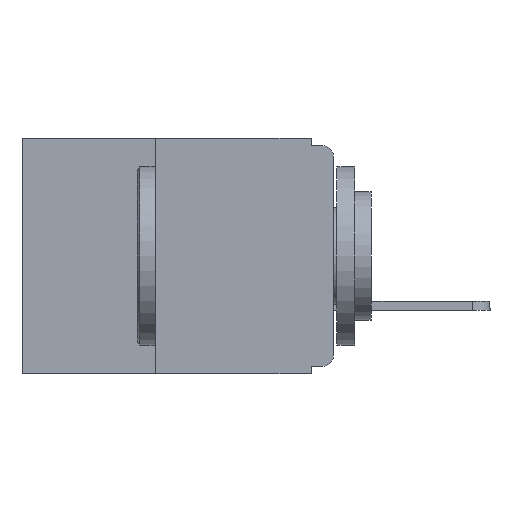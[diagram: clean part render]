
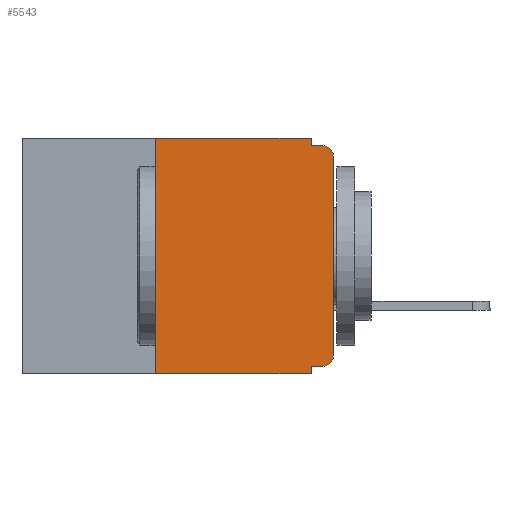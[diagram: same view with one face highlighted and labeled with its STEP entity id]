
A CAD part, left-side view. The second image highlights one B-rep face of the part: STEP entity #5543.
In plain terms, the highlighted planar face has unit normal (-1, 0, 0).
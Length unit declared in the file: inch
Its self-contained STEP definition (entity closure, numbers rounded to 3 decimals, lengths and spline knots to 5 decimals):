
#581 = CARTESIAN_POINT ( 'NONE',  ( 0., 0., -0.01 ) ) ;
#607 = ORIENTED_EDGE ( 'NONE', *, *, #7675, .F. ) ;
#1486 = CIRCLE ( 'NONE', #20408, 0.015 ) ;
#1965 = VERTEX_POINT ( 'NONE', #22940 ) ;
#3889 = EDGE_CURVE ( 'NONE', #5948, #25609, #24349, .T. ) ;
#3914 = VERTEX_POINT ( 'NONE', #12254 ) ;
#4570 = VECTOR ( 'NONE', #22869, 39.37008 ) ;
#5026 = ORIENTED_EDGE ( 'NONE', *, *, #3889, .T. ) ;
#5129 = VECTOR ( 'NONE', #27312, 39.37008 ) ;
#5446 = LINE ( 'NONE', #22341, #30824 ) ;
#5543 = ADVANCED_FACE ( 'NONE', ( #25008 ), #30338, .F. ) ;
#5695 = LINE ( 'NONE', #24946, #18408 ) ;
#5948 = VERTEX_POINT ( 'NONE', #23680 ) ;
#7675 = EDGE_CURVE ( 'NONE', #1965, #3914, #5446, .T. ) ;
#7689 = ORIENTED_EDGE ( 'NONE', *, *, #21768, .T. ) ;
#7765 = AXIS2_PLACEMENT_3D ( 'NONE', #12557, #12517, #12456 ) ;
#7871 = VERTEX_POINT ( 'NONE', #13328 ) ;
#8416 = EDGE_CURVE ( 'NONE', #21649, #16186, #1486, .T. ) ;
#8884 = ORIENTED_EDGE ( 'NONE', *, *, #19534, .F. ) ;
#9687 = DIRECTION ( 'NONE',  ( 0., 0., 1. ) ) ;
#11075 = EDGE_CURVE ( 'NONE', #26376, #20987, #31018, .T. ) ;
#11101 = VECTOR ( 'NONE', #28595, 39.37008 ) ;
#11123 = EDGE_CURVE ( 'NONE', #26376, #12468, #17554, .T. ) ;
#11236 = ORIENTED_EDGE ( 'NONE', *, *, #8416, .T. ) ;
#11551 = VECTOR ( 'NONE', #9687, 39.37008 ) ;
#12254 = CARTESIAN_POINT ( 'NONE',  ( 0., 0.031, -0.01 ) ) ;
#12362 = CARTESIAN_POINT ( 'NONE',  ( 0., 0.25, -0.33 ) ) ;
#12456 = DIRECTION ( 'NONE',  ( 0., 0., -1. ) ) ;
#12468 = VERTEX_POINT ( 'NONE', #23386 ) ;
#12517 = DIRECTION ( 'NONE',  ( -1., 0., 0. ) ) ;
#12557 = CARTESIAN_POINT ( 'NONE',  ( 0., 0.015, -0.305 ) ) ;
#13328 = CARTESIAN_POINT ( 'NONE',  ( 0., 0.031, -0.32 ) ) ;
#14211 = EDGE_LOOP ( 'NONE', ( #7689, #11236, #18025, #607, #8884, #30733, #24819, #15250, #26423, #5026 ) ) ;
#14483 = EDGE_CURVE ( 'NONE', #5948, #7871, #5695, .T. ) ;
#15250 = ORIENTED_EDGE ( 'NONE', *, *, #18009, .F. ) ;
#16186 = VERTEX_POINT ( 'NONE', #29614 ) ;
#17554 = LINE ( 'NONE', #32601, #22709 ) ;
#17883 = LINE ( 'NONE', #581, #11101 ) ;
#18009 = EDGE_CURVE ( 'NONE', #7871, #12468, #32035, .T. ) ;
#18025 = ORIENTED_EDGE ( 'NONE', *, *, #23839, .F. ) ;
#18379 = DIRECTION ( 'NONE',  ( 0., -1., 0. ) ) ;
#18408 = VECTOR ( 'NONE', #27483, 39.37008 ) ;
#19534 = EDGE_CURVE ( 'NONE', #20987, #1965, #32430, .T. ) ;
#20408 = AXIS2_PLACEMENT_3D ( 'NONE', #28085, #28046, #28012 ) ;
#20987 = VERTEX_POINT ( 'NONE', #24174 ) ;
#21649 = VERTEX_POINT ( 'NONE', #29941 ) ;
#21768 = EDGE_CURVE ( 'NONE', #25609, #21649, #29918, .T. ) ;
#22341 = CARTESIAN_POINT ( 'NONE',  ( 0., 0.031, 0. ) ) ;
#22709 = VECTOR ( 'NONE', #30097, 39.37008 ) ;
#22869 = DIRECTION ( 'NONE',  ( 0., 0., 1. ) ) ;
#22940 = CARTESIAN_POINT ( 'NONE',  ( 0., 0.031, 0. ) ) ;
#23385 = DIRECTION ( 'NONE',  ( 0., 0., -1. ) ) ;
#23386 = CARTESIAN_POINT ( 'NONE',  ( 0., 0.031, -0.33 ) ) ;
#23680 = CARTESIAN_POINT ( 'NONE',  ( 0., 0.015, -0.32 ) ) ;
#23839 = EDGE_CURVE ( 'NONE', #3914, #16186, #17883, .T. ) ;
#24174 = CARTESIAN_POINT ( 'NONE',  ( 0., 0.25, 0. ) ) ;
#24349 = CIRCLE ( 'NONE', #7765, 0.015 ) ;
#24538 = CARTESIAN_POINT ( 'NONE',  ( 0., 0., -0.305 ) ) ;
#24778 = CARTESIAN_POINT ( 'NONE',  ( 0., 0.031, -0.33 ) ) ;
#24819 = ORIENTED_EDGE ( 'NONE', *, *, #11123, .T. ) ;
#24946 = CARTESIAN_POINT ( 'NONE',  ( 0., 0., -0.32 ) ) ;
#25008 = FACE_OUTER_BOUND ( 'NONE', #14211, .T. ) ;
#25609 = VERTEX_POINT ( 'NONE', #24538 ) ;
#25736 = VECTOR ( 'NONE', #18379, 39.37008 ) ;
#26376 = VERTEX_POINT ( 'NONE', #12362 ) ;
#26423 = ORIENTED_EDGE ( 'NONE', *, *, #14483, .F. ) ;
#27312 = DIRECTION ( 'NONE',  ( 0., 0., -1. ) ) ;
#27483 = DIRECTION ( 'NONE',  ( 0., 1., 0. ) ) ;
#28012 = DIRECTION ( 'NONE',  ( 0., 0., -1. ) ) ;
#28046 = DIRECTION ( 'NONE',  ( -1., 0., 0. ) ) ;
#28085 = CARTESIAN_POINT ( 'NONE',  ( 0., 0.015, -0.025 ) ) ;
#28457 = CARTESIAN_POINT ( 'NONE',  ( 0., 0.437, 0. ) ) ;
#28595 = DIRECTION ( 'NONE',  ( 0., -1., 0. ) ) ;
#29614 = CARTESIAN_POINT ( 'NONE',  ( 0., 0.015, -0.01 ) ) ;
#29918 = LINE ( 'NONE', #30496, #4570 ) ;
#29941 = CARTESIAN_POINT ( 'NONE',  ( 0., 0., -0.025 ) ) ;
#29981 = CARTESIAN_POINT ( 'NONE',  ( 0., 0.25, -0.33 ) ) ;
#30086 = AXIS2_PLACEMENT_3D ( 'NONE', #30299, #30271, #30263 ) ;
#30097 = DIRECTION ( 'NONE',  ( 0., -1., 0. ) ) ;
#30263 = DIRECTION ( 'NONE',  ( 0., 0., -1. ) ) ;
#30271 = DIRECTION ( 'NONE',  ( 1., 0., 0. ) ) ;
#30299 = CARTESIAN_POINT ( 'NONE',  ( 0., 0.437, 0. ) ) ;
#30338 = PLANE ( 'NONE',  #30086 ) ;
#30496 = CARTESIAN_POINT ( 'NONE',  ( 0., 0., 0. ) ) ;
#30733 = ORIENTED_EDGE ( 'NONE', *, *, #11075, .F. ) ;
#30824 = VECTOR ( 'NONE', #23385, 39.37008 ) ;
#31018 = LINE ( 'NONE', #29981, #11551 ) ;
#32035 = LINE ( 'NONE', #24778, #5129 ) ;
#32430 = LINE ( 'NONE', #28457, #25736 ) ;
#32601 = CARTESIAN_POINT ( 'NONE',  ( 0., 0.437, -0.33 ) ) ;
